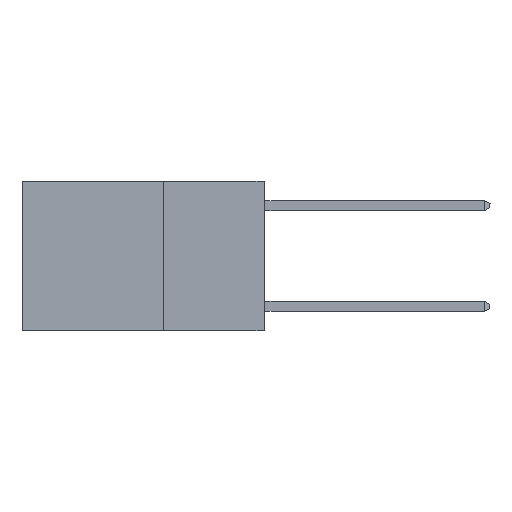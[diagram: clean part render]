
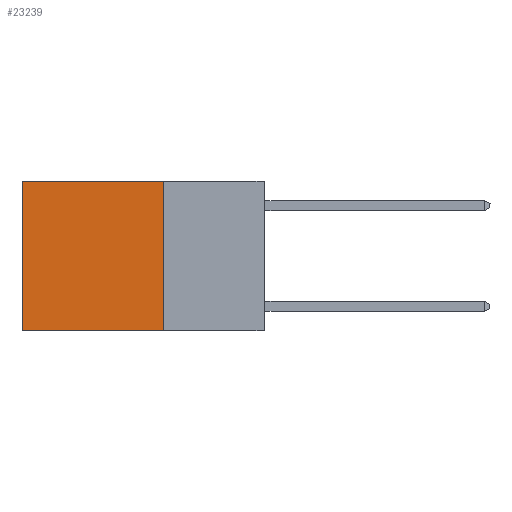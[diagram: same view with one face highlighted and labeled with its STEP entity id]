
A CAD part, left-side view. The second image highlights one B-rep face of the part: STEP entity #23239.
In plain terms, the highlighted planar face has unit normal (-1, 0, 0).
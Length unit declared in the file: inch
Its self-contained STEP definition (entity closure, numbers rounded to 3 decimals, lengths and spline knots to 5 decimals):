
#2897 = FACE_OUTER_BOUND ( 'NONE', #9445, .T. ) ;
#3430 = DIRECTION ( 'NONE',  ( 0., 0., -1. ) ) ;
#3948 = EDGE_CURVE ( 'NONE', #27300, #10270, #15180, .T. ) ;
#5925 = VECTOR ( 'NONE', #3430, 39.37008 ) ;
#7952 = CARTESIAN_POINT ( 'NONE',  ( 0.2625, 0.6, 0. ) ) ;
#9445 = EDGE_LOOP ( 'NONE', ( #18068, #25100, #17641, #25261 ) ) ;
#10270 = VERTEX_POINT ( 'NONE', #22875 ) ;
#11777 = VECTOR ( 'NONE', #24750, 39.37008 ) ;
#13644 = VERTEX_POINT ( 'NONE', #21476 ) ;
#13919 = VECTOR ( 'NONE', #26734, 39.37008 ) ;
#14482 = CARTESIAN_POINT ( 'NONE',  ( 0.2625, 0.6, 0. ) ) ;
#15180 = LINE ( 'NONE', #7952, #11777 ) ;
#15529 = CARTESIAN_POINT ( 'NONE',  ( 0.2625, 0.25, -0.37 ) ) ;
#16703 = EDGE_CURVE ( 'NONE', #22762, #27300, #21877, .T. ) ;
#17163 = CARTESIAN_POINT ( 'NONE',  ( 0.2625, 0.25, 0. ) ) ;
#17641 = ORIENTED_EDGE ( 'NONE', *, *, #29346, .F. ) ;
#17656 = DIRECTION ( 'NONE',  ( 1., 0., 0. ) ) ;
#18068 = ORIENTED_EDGE ( 'NONE', *, *, #3948, .T. ) ;
#19856 = PLANE ( 'NONE',  #25178 ) ;
#20016 = CARTESIAN_POINT ( 'NONE',  ( 0.2625, 0.25, 0. ) ) ;
#21476 = CARTESIAN_POINT ( 'NONE',  ( 0.2625, 0.25, -0.37 ) ) ;
#21658 = CARTESIAN_POINT ( 'NONE',  ( 0.2625, 0.25, 0. ) ) ;
#21877 = LINE ( 'NONE', #17163, #13919 ) ;
#22762 = VERTEX_POINT ( 'NONE', #21658 ) ;
#22875 = CARTESIAN_POINT ( 'NONE',  ( 0.2625, 0.6, -0.37 ) ) ;
#23239 = ADVANCED_FACE ( 'NONE', ( #2897 ), #19856, .F. ) ;
#24516 = EDGE_CURVE ( 'NONE', #13644, #10270, #28534, .T. ) ;
#24750 = DIRECTION ( 'NONE',  ( 0., 0., -1. ) ) ;
#24943 = LINE ( 'NONE', #30136, #5925 ) ;
#25100 = ORIENTED_EDGE ( 'NONE', *, *, #24516, .F. ) ;
#25178 = AXIS2_PLACEMENT_3D ( 'NONE', #20016, #17656, #29432 ) ;
#25261 = ORIENTED_EDGE ( 'NONE', *, *, #16703, .T. ) ;
#26469 = DIRECTION ( 'NONE',  ( 0., 1., 0. ) ) ;
#26734 = DIRECTION ( 'NONE',  ( 0., 1., 0. ) ) ;
#27300 = VERTEX_POINT ( 'NONE', #14482 ) ;
#28534 = LINE ( 'NONE', #15529, #30237 ) ;
#29346 = EDGE_CURVE ( 'NONE', #22762, #13644, #24943, .T. ) ;
#29432 = DIRECTION ( 'NONE',  ( 0., 0., -1. ) ) ;
#30136 = CARTESIAN_POINT ( 'NONE',  ( 0.2625, 0.25, 0. ) ) ;
#30237 = VECTOR ( 'NONE', #26469, 39.37008 ) ;
